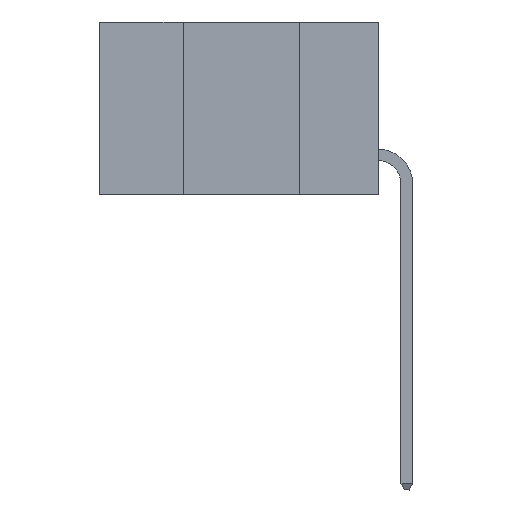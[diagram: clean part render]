
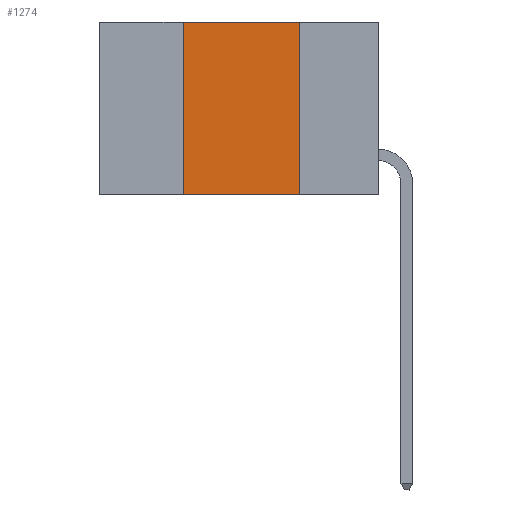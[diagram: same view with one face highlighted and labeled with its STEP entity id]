
A CAD part, left-side view. The second image highlights one B-rep face of the part: STEP entity #1274.
In plain terms, the highlighted planar face has unit normal (-1, 0, 0).
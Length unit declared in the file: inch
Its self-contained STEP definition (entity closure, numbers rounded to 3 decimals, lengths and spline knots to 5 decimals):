
#164 = DIRECTION ( 'NONE',  ( 0., 0., 1. ) ) ;
#526 = VERTEX_POINT ( 'NONE', #12746 ) ;
#1245 = LINE ( 'NONE', #1482, #4168 ) ;
#1274 = ADVANCED_FACE ( 'NONE', ( #13397 ), #10089, .F. ) ;
#1482 = CARTESIAN_POINT ( 'NONE',  ( 0., 0.6, 0. ) ) ;
#1539 = CARTESIAN_POINT ( 'NONE',  ( 0., 0.6, 0. ) ) ;
#3375 = CARTESIAN_POINT ( 'NONE',  ( 0., 0.17, 0. ) ) ;
#3934 = VERTEX_POINT ( 'NONE', #17078 ) ;
#4168 = VECTOR ( 'NONE', #7576, 39.37008 ) ;
#4945 = CARTESIAN_POINT ( 'NONE',  ( 0., 0.42, -0.37 ) ) ;
#5407 = EDGE_CURVE ( 'NONE', #6977, #16496, #12664, .T. ) ;
#6210 = VECTOR ( 'NONE', #10587, 39.37008 ) ;
#6357 = EDGE_CURVE ( 'NONE', #526, #3934, #12381, .T. ) ;
#6977 = VERTEX_POINT ( 'NONE', #4945 ) ;
#7002 = CARTESIAN_POINT ( 'NONE',  ( 0., 0.42, 0. ) ) ;
#7334 = VECTOR ( 'NONE', #13545, 39.37008 ) ;
#7576 = DIRECTION ( 'NONE',  ( 0., -1., 0. ) ) ;
#8314 = EDGE_CURVE ( 'NONE', #16496, #526, #1245, .T. ) ;
#9460 = EDGE_LOOP ( 'NONE', ( #17298, #9631, #11881, #17396 ) ) ;
#9631 = ORIENTED_EDGE ( 'NONE', *, *, #8314, .F. ) ;
#10089 = PLANE ( 'NONE',  #17991 ) ;
#10587 = DIRECTION ( 'NONE',  ( 0., 0., -1. ) ) ;
#10800 = CARTESIAN_POINT ( 'NONE',  ( 0., 0.42, 0. ) ) ;
#11119 = LINE ( 'NONE', #13481, #7334 ) ;
#11335 = VECTOR ( 'NONE', #164, 39.37008 ) ;
#11881 = ORIENTED_EDGE ( 'NONE', *, *, #5407, .F. ) ;
#12381 = LINE ( 'NONE', #3375, #6210 ) ;
#12664 = LINE ( 'NONE', #7002, #11335 ) ;
#12746 = CARTESIAN_POINT ( 'NONE',  ( 0., 0.17, 0. ) ) ;
#13397 = FACE_OUTER_BOUND ( 'NONE', #9460, .T. ) ;
#13481 = CARTESIAN_POINT ( 'NONE',  ( 0., 0.6, -0.37 ) ) ;
#13545 = DIRECTION ( 'NONE',  ( 0., -1., 0. ) ) ;
#14172 = EDGE_CURVE ( 'NONE', #6977, #3934, #11119, .T. ) ;
#14281 = DIRECTION ( 'NONE',  ( 1., 0., 0. ) ) ;
#15841 = DIRECTION ( 'NONE',  ( 0., 0., -1. ) ) ;
#16496 = VERTEX_POINT ( 'NONE', #10800 ) ;
#17078 = CARTESIAN_POINT ( 'NONE',  ( 0., 0.17, -0.37 ) ) ;
#17298 = ORIENTED_EDGE ( 'NONE', *, *, #6357, .F. ) ;
#17396 = ORIENTED_EDGE ( 'NONE', *, *, #14172, .T. ) ;
#17991 = AXIS2_PLACEMENT_3D ( 'NONE', #1539, #14281, #15841 ) ;
